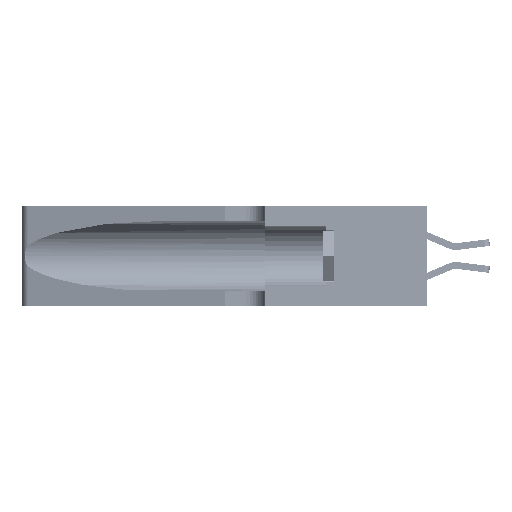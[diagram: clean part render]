
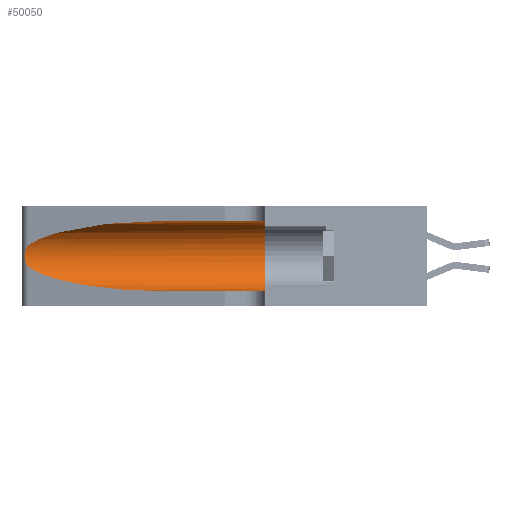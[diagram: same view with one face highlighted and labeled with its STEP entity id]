
A CAD part, left-side view. The second image highlights one B-rep face of the part: STEP entity #50050.
In plain terms, the highlighted cylindrical face has radius 3.308 mm (diameter 6.617 mm), a partial arc.
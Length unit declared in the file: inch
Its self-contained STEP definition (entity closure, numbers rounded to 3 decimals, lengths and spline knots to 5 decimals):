
#675 = CARTESIAN_POINT ( 'NONE',  ( 0.26017, 1.23833, 0.17102 ) ) ;
#887 = VERTEX_POINT ( 'NONE', #31843 ) ;
#1272 = CYLINDRICAL_SURFACE ( 'NONE', #30225, 0.13025 ) ;
#1294 = ORIENTED_EDGE ( 'NONE', *, *, #38382, .F. ) ;
#3801 = CARTESIAN_POINT ( 'NONE',  ( 0.1305, 0.72297, 0.31525 ) ) ;
#4166 = EDGE_CURVE ( 'NONE', #35130, #50769, #11752, .T. ) ;
#5049 = CARTESIAN_POINT ( 'NONE',  ( 0.25555, 1.22994, 0.2215 ) ) ;
#5586 = CARTESIAN_POINT ( 'NONE',  ( 0.1305, 0.35, 0.185 ) ) ;
#7147 = CARTESIAN_POINT ( 'NONE',  ( 0.25487, 1.22718, 0.22369 ) ) ;
#7714 = ORIENTED_EDGE ( 'NONE', *, *, #29220, .T. ) ;
#8071 = EDGE_LOOP ( 'NONE', ( #21528, #42546, #25371, #7714, #1294, #34806 ) ) ;
#8145 = FACE_OUTER_BOUND ( 'NONE', #8071, .T. ) ;
#8335 = CARTESIAN_POINT ( 'NONE',  ( 0.25487, 1.22718, 0.22369 ) ) ;
#8725 = CARTESIAN_POINT ( 'NONE',  ( 0.25487, 1.22718, 0.22369 ) ) ;
#11752 =( BOUNDED_CURVE ( )  B_SPLINE_CURVE ( 3, ( #39582, #24251, #47933, #32101 ),
 .UNSPECIFIED., .F., .F. ) 
 B_SPLINE_CURVE_WITH_KNOTS ( ( 4, 4 ),
 ( 3.44316, 4.71239 ),
 .UNSPECIFIED. ) 
 CURVE ( )  GEOMETRIC_REPRESENTATION_ITEM ( )  RATIONAL_B_SPLINE_CURVE ( ( 1., 0.87, 0.87, 1. ) ) 
 REPRESENTATION_ITEM ( '' )  );
#12571 = CARTESIAN_POINT ( 'NONE',  ( 0.25639, 1.23184, 0.21858 ) ) ;
#12935 = CARTESIAN_POINT ( 'NONE',  ( 0.26075, 1.23896, 0.178 ) ) ;
#13108 = CARTESIAN_POINT ( 'NONE',  ( 0.26075, 1.23896, 0.19203 ) ) ;
#13800 = DIRECTION ( 'NONE',  ( 0., -1., 0. ) ) ;
#14524 = CIRCLE ( 'NONE', #33845, 0.13025 ) ;
#16079 = CARTESIAN_POINT ( 'NONE',  ( 0.25487, 1.22718, 0.14631 ) ) ;
#17153 = CARTESIAN_POINT ( 'NONE',  ( 0.25555, 1.22993, 0.14849 ) ) ;
#17761 = DIRECTION ( 'NONE',  ( 0., -1., 0. ) ) ;
#21164 = CARTESIAN_POINT ( 'NONE',  ( 0.25487, 1.22718, 0.14631 ) ) ;
#21528 = ORIENTED_EDGE ( 'NONE', *, *, #51249, .T. ) ;
#22255 = VERTEX_POINT ( 'NONE', #7147 ) ;
#23412 = CARTESIAN_POINT ( 'NONE',  ( 0.2373, 1.15595, 0.28018 ) ) ;
#24251 = CARTESIAN_POINT ( 'NONE',  ( 0.2373, 1.15595, 0.08982 ) ) ;
#24476 = CARTESIAN_POINT ( 'NONE',  ( 0.1305, 0.72297, 0.31525 ) ) ;
#25290 = DIRECTION ( 'NONE',  ( 0., 0., -1. ) ) ;
#25371 = ORIENTED_EDGE ( 'NONE', *, *, #4166, .T. ) ;
#27078 = LINE ( 'NONE', #50699, #34498 ) ;
#28671 = CARTESIAN_POINT ( 'NONE',  ( 0.25639, 1.23186, 0.15144 ) ) ;
#29220 = EDGE_CURVE ( 'NONE', #50769, #887, #27078, .T. ) ;
#29716 = CARTESIAN_POINT ( 'NONE',  ( 0.1305, 0.72297, 0.05475 ) ) ;
#30225 = AXIS2_PLACEMENT_3D ( 'NONE', #45275, #17761, #25290 ) ;
#31843 = CARTESIAN_POINT ( 'NONE',  ( 0.1305, 0.35, 0.05475 ) ) ;
#32101 = CARTESIAN_POINT ( 'NONE',  ( 0.1305, 0.72297, 0.05475 ) ) ;
#32655 = CARTESIAN_POINT ( 'NONE',  ( 0.25787, 1.23484, 0.2124 ) ) ;
#33004 = CARTESIAN_POINT ( 'NONE',  ( 0.25856, 1.23593, 0.16098 ) ) ;
#33021 = DIRECTION ( 'NONE',  ( 0., 1., 0. ) ) ;
#33079 = EDGE_CURVE ( 'NONE', #22255, #35130, #35740, .T. ) ;
#33845 = AXIS2_PLACEMENT_3D ( 'NONE', #5586, #33021, #41714 ) ;
#34498 = VECTOR ( 'NONE', #35191, 39.37008 ) ;
#34806 = ORIENTED_EDGE ( 'NONE', *, *, #46550, .F. ) ;
#35130 = VERTEX_POINT ( 'NONE', #16079 ) ;
#35191 = DIRECTION ( 'NONE',  ( 0., -1., 0. ) ) ;
#35278 = VECTOR ( 'NONE', #13800, 39.37008 ) ;
#35740 = B_SPLINE_CURVE_WITH_KNOTS ( 'NONE', 3,
 ( #8725, #5049, #12571, #32655, #36644, #36812, #13108, #12935, #675, #33004, #41004, #28671, #17153, #21164 ),
 .UNSPECIFIED., .F., .F.,
 ( 4, 2, 2, 2, 2, 2, 4 ),
 ( 0., 0.00027, 0.00053, 0.00107, 0.0016, 0.00187, 0.00214 ),
 .UNSPECIFIED. ) ;
#35922 = LINE ( 'NONE', #50009, #35278 ) ;
#36644 = CARTESIAN_POINT ( 'NONE',  ( 0.25854, 1.2359, 0.20912 ) ) ;
#36812 = CARTESIAN_POINT ( 'NONE',  ( 0.26018, 1.23835, 0.19895 ) ) ;
#38382 = EDGE_CURVE ( 'NONE', #41486, #887, #14524, .T. ) ;
#39582 = CARTESIAN_POINT ( 'NONE',  ( 0.25487, 1.22718, 0.14631 ) ) ;
#41004 = CARTESIAN_POINT ( 'NONE',  ( 0.25789, 1.23486, 0.15765 ) ) ;
#41486 = VERTEX_POINT ( 'NONE', #45937 ) ;
#41714 = DIRECTION ( 'NONE',  ( 0., 0., 1. ) ) ;
#41822 =( BOUNDED_CURVE ( )  B_SPLINE_CURVE ( 3, ( #3801, #43776, #23412, #8335 ),
 .UNSPECIFIED., .F., .F. ) 
 B_SPLINE_CURVE_WITH_KNOTS ( ( 4, 4 ),
 ( 1.5708, 2.84003 ),
 .UNSPECIFIED. ) 
 CURVE ( )  GEOMETRIC_REPRESENTATION_ITEM ( )  RATIONAL_B_SPLINE_CURVE ( ( 1., 0.87, 0.87, 1. ) ) 
 REPRESENTATION_ITEM ( '' )  );
#42546 = ORIENTED_EDGE ( 'NONE', *, *, #33079, .T. ) ;
#43776 = CARTESIAN_POINT ( 'NONE',  ( 0.18966, 0.96281, 0.31525 ) ) ;
#44844 = VERTEX_POINT ( 'NONE', #24476 ) ;
#45275 = CARTESIAN_POINT ( 'NONE',  ( 0.1305, 1.61858, 0.185 ) ) ;
#45937 = CARTESIAN_POINT ( 'NONE',  ( 0.1305, 0.35, 0.31525 ) ) ;
#46550 = EDGE_CURVE ( 'NONE', #44844, #41486, #35922, .T. ) ;
#47933 = CARTESIAN_POINT ( 'NONE',  ( 0.18966, 0.96281, 0.05475 ) ) ;
#50009 = CARTESIAN_POINT ( 'NONE',  ( 0.1305, 1.61858, 0.31525 ) ) ;
#50050 = ADVANCED_FACE ( 'NONE', ( #8145 ), #1272, .F. ) ;
#50699 = CARTESIAN_POINT ( 'NONE',  ( 0.1305, 1.61858, 0.05475 ) ) ;
#50769 = VERTEX_POINT ( 'NONE', #29716 ) ;
#51249 = EDGE_CURVE ( 'NONE', #44844, #22255, #41822, .T. ) ;
